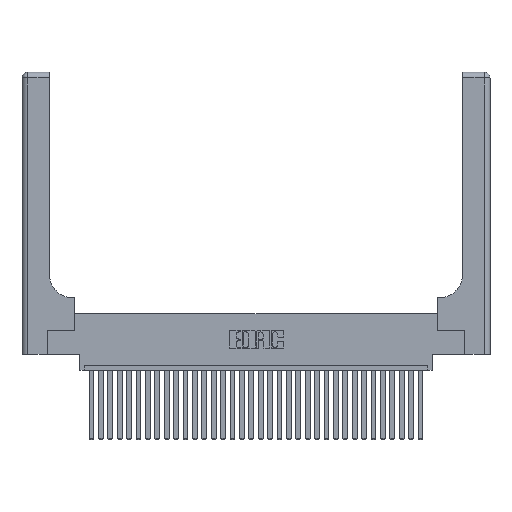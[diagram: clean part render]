
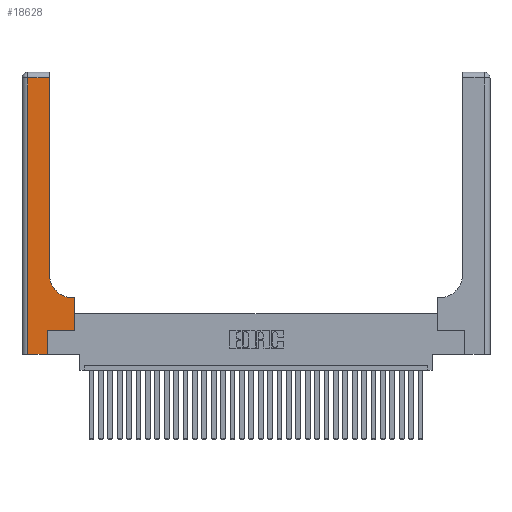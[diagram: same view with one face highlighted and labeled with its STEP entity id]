
A CAD part, top view. The second image highlights one B-rep face of the part: STEP entity #18628.
In plain terms, the highlighted planar face has unit normal (0, 0, 1).
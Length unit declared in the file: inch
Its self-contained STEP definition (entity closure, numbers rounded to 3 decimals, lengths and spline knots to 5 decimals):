
#249 = EDGE_CURVE ( 'NONE', #16942, #9857, #32188, .T. ) ;
#1265 = LINE ( 'NONE', #15437, #23954 ) ;
#1322 = DIRECTION ( 'NONE',  ( -1., 0., 0. ) ) ;
#1863 = VECTOR ( 'NONE', #21004, 39.37008 ) ;
#2237 = ORIENTED_EDGE ( 'NONE', *, *, #27387, .T. ) ;
#2455 = LINE ( 'NONE', #22833, #7241 ) ;
#2482 = DIRECTION ( 'NONE',  ( 1., 0., 0. ) ) ;
#2726 = EDGE_CURVE ( 'NONE', #6188, #18939, #1265, .T. ) ;
#3084 = DIRECTION ( 'NONE',  ( -1., 0., 0. ) ) ;
#3192 = CARTESIAN_POINT ( 'NONE',  ( 0., 3., 0.37 ) ) ;
#4203 = VECTOR ( 'NONE', #1322, 39.37008 ) ;
#4292 = CARTESIAN_POINT ( 'NONE',  ( 0.269, 0., 0.37 ) ) ;
#4839 = DIRECTION ( 'NONE',  ( 0., 1., 0. ) ) ;
#5036 = CARTESIAN_POINT ( 'NONE',  ( 0.5415, 0.6, 0.37 ) ) ;
#5337 = VERTEX_POINT ( 'NONE', #20759 ) ;
#5772 = LINE ( 'NONE', #26729, #4203 ) ;
#6188 = VERTEX_POINT ( 'NONE', #6762 ) ;
#6367 = ORIENTED_EDGE ( 'NONE', *, *, #8515, .T. ) ;
#6650 = ORIENTED_EDGE ( 'NONE', *, *, #15459, .T. ) ;
#6762 = CARTESIAN_POINT ( 'NONE',  ( 0.06, 0., 0.37 ) ) ;
#6846 = ORIENTED_EDGE ( 'NONE', *, *, #13204, .T. ) ;
#7054 = ORIENTED_EDGE ( 'NONE', *, *, #7125, .T. ) ;
#7125 = EDGE_CURVE ( 'NONE', #20369, #6188, #13467, .T. ) ;
#7241 = VECTOR ( 'NONE', #25549, 39.37008 ) ;
#7633 = ORIENTED_EDGE ( 'NONE', *, *, #2726, .T. ) ;
#8257 = DIRECTION ( 'NONE',  ( 1., 0., 0. ) ) ;
#8286 = CARTESIAN_POINT ( 'NONE',  ( 0.269, 0.25, 0.37 ) ) ;
#8515 = EDGE_CURVE ( 'NONE', #9270, #20369, #5772, .T. ) ;
#8713 = VECTOR ( 'NONE', #23921, 39.37008 ) ;
#9116 = ORIENTED_EDGE ( 'NONE', *, *, #11129, .T. ) ;
#9270 = VERTEX_POINT ( 'NONE', #32263 ) ;
#9756 = DIRECTION ( 'NONE',  ( 1., 0., 0. ) ) ;
#9857 = VERTEX_POINT ( 'NONE', #32893 ) ;
#10864 = LINE ( 'NONE', #12787, #13226 ) ;
#11129 = EDGE_CURVE ( 'NONE', #9857, #9270, #10864, .T. ) ;
#11233 = VECTOR ( 'NONE', #20945, 39.37008 ) ;
#12787 = CARTESIAN_POINT ( 'NONE',  ( 0.2915, 3., 0.37 ) ) ;
#13204 = EDGE_CURVE ( 'NONE', #31609, #5337, #31520, .T. ) ;
#13226 = VECTOR ( 'NONE', #4839, 39.37008 ) ;
#13364 = DIRECTION ( 'NONE',  ( 0., 0., -1. ) ) ;
#13467 = LINE ( 'NONE', #20784, #1863 ) ;
#13608 = CARTESIAN_POINT ( 'NONE',  ( 0.5585, 0.6, 0.37 ) ) ;
#14868 = CARTESIAN_POINT ( 'NONE',  ( 0.5415, 0.85, 0.37 ) ) ;
#15437 = CARTESIAN_POINT ( 'NONE',  ( 0., 0., 0.37 ) ) ;
#15459 = EDGE_CURVE ( 'NONE', #5337, #15833, #31821, .T. ) ;
#15627 = AXIS2_PLACEMENT_3D ( 'NONE', #14868, #19860, #9756 ) ;
#15833 = VERTEX_POINT ( 'NONE', #13608 ) ;
#16942 = VERTEX_POINT ( 'NONE', #5036 ) ;
#18307 = AXIS2_PLACEMENT_3D ( 'NONE', #3192, #13364, #3084 ) ;
#18628 = ADVANCED_FACE ( 'NONE', ( #29399 ), #23872, .F. ) ;
#18939 = VERTEX_POINT ( 'NONE', #4292 ) ;
#19133 = LINE ( 'NONE', #28634, #11233 ) ;
#19807 = EDGE_CURVE ( 'NONE', #15833, #16942, #19133, .T. ) ;
#19860 = DIRECTION ( 'NONE',  ( 0., 0., -1. ) ) ;
#20369 = VERTEX_POINT ( 'NONE', #31059 ) ;
#20759 = CARTESIAN_POINT ( 'NONE',  ( 0.5585, 0.25, 0.37 ) ) ;
#20784 = CARTESIAN_POINT ( 'NONE',  ( 0.06, 3., 0.37 ) ) ;
#20945 = DIRECTION ( 'NONE',  ( -1., 0., 0. ) ) ;
#21004 = DIRECTION ( 'NONE',  ( 0., -1., 0. ) ) ;
#21144 = VECTOR ( 'NONE', #8257, 39.37008 ) ;
#22833 = CARTESIAN_POINT ( 'NONE',  ( 0.269, 0., 0.37 ) ) ;
#22965 = ORIENTED_EDGE ( 'NONE', *, *, #249, .T. ) ;
#23872 = PLANE ( 'NONE',  #18307 ) ;
#23921 = DIRECTION ( 'NONE',  ( 0., 1., 0. ) ) ;
#23954 = VECTOR ( 'NONE', #2482, 39.37008 ) ;
#25192 = ORIENTED_EDGE ( 'NONE', *, *, #19807, .T. ) ;
#25549 = DIRECTION ( 'NONE',  ( 0., 1., 0. ) ) ;
#26076 = CARTESIAN_POINT ( 'NONE',  ( 0.269, 0.25, 0.37 ) ) ;
#26536 = CARTESIAN_POINT ( 'NONE',  ( 0.5585, 0.25, 0.37 ) ) ;
#26729 = CARTESIAN_POINT ( 'NONE',  ( 0., 2.94, 0.37 ) ) ;
#27387 = EDGE_CURVE ( 'NONE', #18939, #31609, #2455, .T. ) ;
#28634 = CARTESIAN_POINT ( 'NONE',  ( 0.2915, 0.6, 0.37 ) ) ;
#28964 = EDGE_LOOP ( 'NONE', ( #9116, #6367, #7054, #7633, #2237, #6846, #6650, #25192, #22965 ) ) ;
#29399 = FACE_OUTER_BOUND ( 'NONE', #28964, .T. ) ;
#31059 = CARTESIAN_POINT ( 'NONE',  ( 0.06, 2.94, 0.37 ) ) ;
#31520 = LINE ( 'NONE', #26076, #21144 ) ;
#31609 = VERTEX_POINT ( 'NONE', #8286 ) ;
#31821 = LINE ( 'NONE', #26536, #8713 ) ;
#32188 = CIRCLE ( 'NONE', #15627, 0.25 ) ;
#32263 = CARTESIAN_POINT ( 'NONE',  ( 0.2915, 2.94, 0.37 ) ) ;
#32893 = CARTESIAN_POINT ( 'NONE',  ( 0.2915, 0.85, 0.37 ) ) ;
